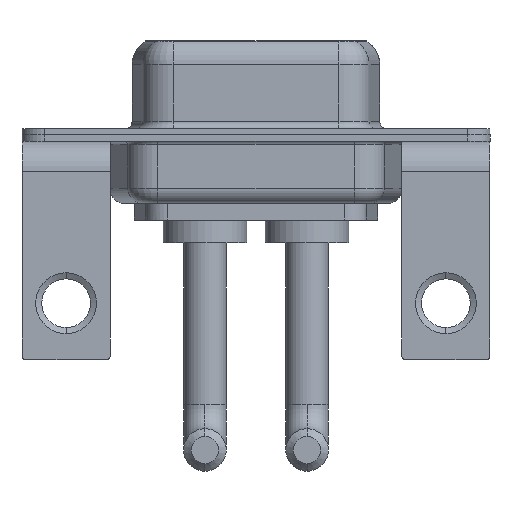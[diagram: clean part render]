
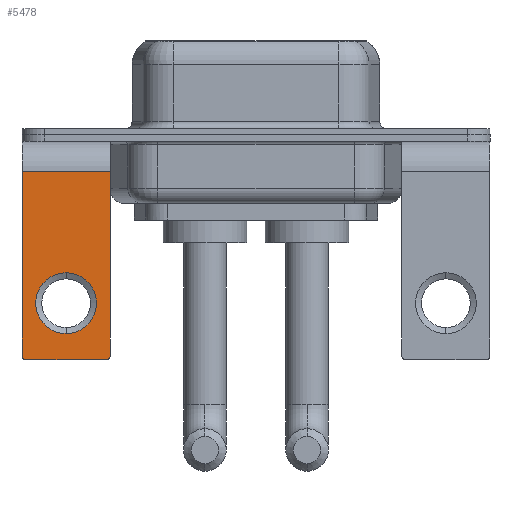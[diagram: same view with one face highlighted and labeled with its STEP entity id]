
A CAD part, front view. The second image highlights one B-rep face of the part: STEP entity #5478.
In plain terms, the highlighted planar face has unit normal (0, -1, 0).
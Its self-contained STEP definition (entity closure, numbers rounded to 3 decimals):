
#83 = ORIENTED_EDGE ( 'NONE', *, *, #7048, .T. ) ;
#346 = VECTOR ( 'NONE', #1079, 1000. ) ;
#568 = CARTESIAN_POINT ( 'NONE',  ( 0., -6.25, -9.07 ) ) ;
#1079 = DIRECTION ( 'NONE',  ( 0., 0., -1. ) ) ;
#1327 = ORIENTED_EDGE ( 'NONE', *, *, #2714, .T. ) ;
#1387 = DIRECTION ( 'NONE',  ( 0., 1., 0. ) ) ;
#1935 = ORIENTED_EDGE ( 'NONE', *, *, #9613, .F. ) ;
#1967 = PLANE ( 'NONE',  #9344 ) ;
#2092 = CARTESIAN_POINT ( 'NONE',  ( 2.9, -6.25, -14.8 ) ) ;
#2150 = DIRECTION ( 'NONE',  ( -1., 0., 0. ) ) ;
#2435 = CARTESIAN_POINT ( 'NONE',  ( 2.65, -6.25, -14.8 ) ) ;
#2445 = DIRECTION ( 'NONE',  ( -1., 0., 0. ) ) ;
#2714 = EDGE_CURVE ( 'NONE', #3641, #6370, #8231, .T. ) ;
#2741 = VERTEX_POINT ( 'NONE', #2435 ) ;
#2763 = CARTESIAN_POINT ( 'NONE',  ( -2.9, -6.25, -2.4 ) ) ;
#3041 = CARTESIAN_POINT ( 'NONE',  ( 0., -6.25, -11.07 ) ) ;
#3073 = ORIENTED_EDGE ( 'NONE', *, *, #5957, .T. ) ;
#3311 = DIRECTION ( 'NONE',  ( 0., -1., 0. ) ) ;
#3641 = VERTEX_POINT ( 'NONE', #3763 ) ;
#3752 = EDGE_CURVE ( 'NONE', #6585, #7293, #8488, .T. ) ;
#3763 = CARTESIAN_POINT ( 'NONE',  ( -2.9, -6.25, -14.55 ) ) ;
#3805 = AXIS2_PLACEMENT_3D ( 'NONE', #12277, #3311, #11289 ) ;
#4236 = CARTESIAN_POINT ( 'NONE',  ( -2.9, -6.25, -2.4 ) ) ;
#4238 = CARTESIAN_POINT ( 'NONE',  ( 2.9, -6.25, -2.4 ) ) ;
#4393 = CARTESIAN_POINT ( 'NONE',  ( 2.9, -6.25, -14.55 ) ) ;
#4624 = ORIENTED_EDGE ( 'NONE', *, *, #11661, .T. ) ;
#4635 = EDGE_CURVE ( 'NONE', #2741, #4767, #7968, .T. ) ;
#4767 = VERTEX_POINT ( 'NONE', #4393 ) ;
#5134 = VECTOR ( 'NONE', #2150, 1000. ) ;
#5163 = DIRECTION ( 'NONE',  ( 0., 0., 1. ) ) ;
#5446 = VERTEX_POINT ( 'NONE', #12051 ) ;
#5478 = ADVANCED_FACE ( 'NONE', ( #7120, #10141 ), #1967, .F. ) ;
#5625 = CARTESIAN_POINT ( 'NONE',  ( -2.65, -6.25, -14.55 ) ) ;
#5635 = LINE ( 'NONE', #12654, #10831 ) ;
#5779 = LINE ( 'NONE', #12921, #346 ) ;
#5818 = DIRECTION ( 'NONE',  ( 0., 0., -1. ) ) ;
#5957 = EDGE_CURVE ( 'NONE', #5446, #12176, #5635, .T. ) ;
#6336 = CARTESIAN_POINT ( 'NONE',  ( 0., -6.25, -11.07 ) ) ;
#6370 = VERTEX_POINT ( 'NONE', #10921 ) ;
#6585 = VERTEX_POINT ( 'NONE', #568 ) ;
#6699 = EDGE_LOOP ( 'NONE', ( #83, #1327, #12650, #10338, #1935, #3073 ) ) ;
#7048 = EDGE_CURVE ( 'NONE', #12176, #3641, #11732, .T. ) ;
#7120 = FACE_BOUND ( 'NONE', #9573, .T. ) ;
#7293 = VERTEX_POINT ( 'NONE', #10400 ) ;
#7968 = CIRCLE ( 'NONE', #3805, 0.25 ) ;
#7993 = DIRECTION ( 'NONE',  ( 0., 1., 0. ) ) ;
#8161 = DIRECTION ( 'NONE',  ( 0., 0., 1. ) ) ;
#8231 = CIRCLE ( 'NONE', #8867, 0.25 ) ;
#8488 = CIRCLE ( 'NONE', #11853, 2. ) ;
#8867 = AXIS2_PLACEMENT_3D ( 'NONE', #5625, #10488, #9638 ) ;
#9023 = EDGE_CURVE ( 'NONE', #2741, #6370, #12109, .T. ) ;
#9079 = ORIENTED_EDGE ( 'NONE', *, *, #3752, .T. ) ;
#9207 = VECTOR ( 'NONE', #5818, 1000. ) ;
#9265 = CIRCLE ( 'NONE', #10528, 2. ) ;
#9344 = AXIS2_PLACEMENT_3D ( 'NONE', #4238, #10997, #8161 ) ;
#9573 = EDGE_LOOP ( 'NONE', ( #4624, #9079 ) ) ;
#9613 = EDGE_CURVE ( 'NONE', #5446, #4767, #5779, .T. ) ;
#9638 = DIRECTION ( 'NONE',  ( 0., 0., 1. ) ) ;
#10035 = DIRECTION ( 'NONE',  ( 0., 0., 1. ) ) ;
#10141 = FACE_OUTER_BOUND ( 'NONE', #6699, .T. ) ;
#10338 = ORIENTED_EDGE ( 'NONE', *, *, #4635, .T. ) ;
#10400 = CARTESIAN_POINT ( 'NONE',  ( 0., -6.25, -13.07 ) ) ;
#10488 = DIRECTION ( 'NONE',  ( 0., -1., 0. ) ) ;
#10528 = AXIS2_PLACEMENT_3D ( 'NONE', #6336, #1387, #5163 ) ;
#10831 = VECTOR ( 'NONE', #2445, 1000. ) ;
#10921 = CARTESIAN_POINT ( 'NONE',  ( -2.65, -6.25, -14.8 ) ) ;
#10997 = DIRECTION ( 'NONE',  ( 0., 1., 0. ) ) ;
#11289 = DIRECTION ( 'NONE',  ( 0., 0., 1. ) ) ;
#11661 = EDGE_CURVE ( 'NONE', #7293, #6585, #9265, .T. ) ;
#11732 = LINE ( 'NONE', #2763, #9207 ) ;
#11853 = AXIS2_PLACEMENT_3D ( 'NONE', #3041, #7993, #10035 ) ;
#12051 = CARTESIAN_POINT ( 'NONE',  ( 2.9, -6.25, -2.4 ) ) ;
#12109 = LINE ( 'NONE', #2092, #5134 ) ;
#12176 = VERTEX_POINT ( 'NONE', #4236 ) ;
#12277 = CARTESIAN_POINT ( 'NONE',  ( 2.65, -6.25, -14.55 ) ) ;
#12650 = ORIENTED_EDGE ( 'NONE', *, *, #9023, .F. ) ;
#12654 = CARTESIAN_POINT ( 'NONE',  ( 2.9, -6.25, -2.4 ) ) ;
#12921 = CARTESIAN_POINT ( 'NONE',  ( 2.9, -6.25, -2.4 ) ) ;
